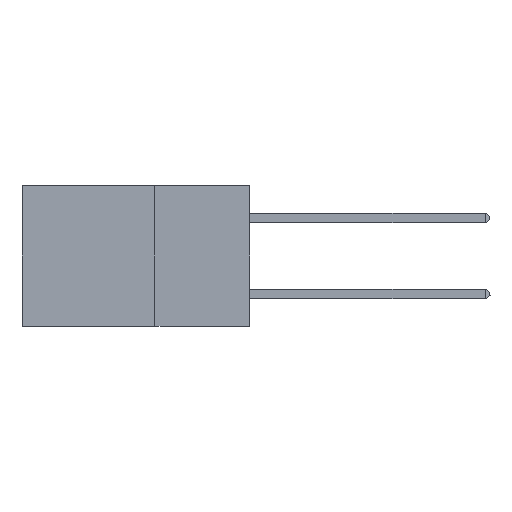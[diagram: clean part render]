
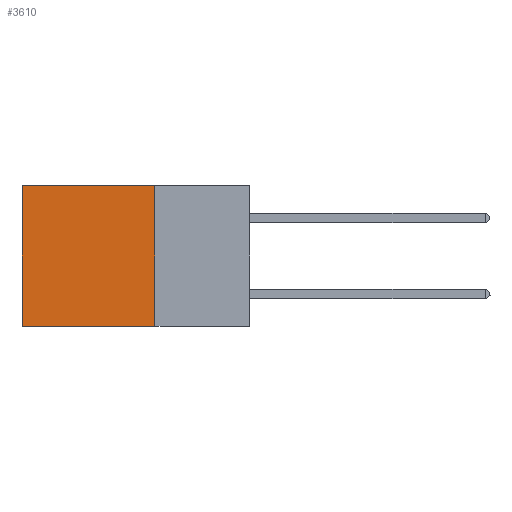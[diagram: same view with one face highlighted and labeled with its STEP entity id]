
A CAD part, left-side view. The second image highlights one B-rep face of the part: STEP entity #3610.
In plain terms, the highlighted planar face has unit normal (-1, 0, 0).
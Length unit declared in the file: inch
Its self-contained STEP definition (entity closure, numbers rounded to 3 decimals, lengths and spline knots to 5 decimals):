
#466 = CARTESIAN_POINT ( 'NONE',  ( 0.2875, 0.25, 0. ) ) ;
#864 = CARTESIAN_POINT ( 'NONE',  ( 0.2875, 0.25, 0. ) ) ;
#1117 = VECTOR ( 'NONE', #8852, 39.37008 ) ;
#1227 = CARTESIAN_POINT ( 'NONE',  ( 0.2875, 0.25, 0. ) ) ;
#1508 = DIRECTION ( 'NONE',  ( 0., 0., -1. ) ) ;
#2467 = VERTEX_POINT ( 'NONE', #14720 ) ;
#3610 = ADVANCED_FACE ( 'NONE', ( #17761 ), #21781, .F. ) ;
#3894 = VECTOR ( 'NONE', #4807, 39.37008 ) ;
#4807 = DIRECTION ( 'NONE',  ( 0., 1., 0. ) ) ;
#6198 = DIRECTION ( 'NONE',  ( 0., 0., -1. ) ) ;
#6285 = LINE ( 'NONE', #6545, #14133 ) ;
#6545 = CARTESIAN_POINT ( 'NONE',  ( 0.2875, 0.6, 0. ) ) ;
#7256 = ORIENTED_EDGE ( 'NONE', *, *, #13277, .T. ) ;
#7293 = VERTEX_POINT ( 'NONE', #466 ) ;
#8146 = ORIENTED_EDGE ( 'NONE', *, *, #11430, .F. ) ;
#8852 = DIRECTION ( 'NONE',  ( 0., 1., 0. ) ) ;
#9520 = ORIENTED_EDGE ( 'NONE', *, *, #18389, .F. ) ;
#9858 = CARTESIAN_POINT ( 'NONE',  ( 0.2875, 0.25, -0.37 ) ) ;
#10130 = VECTOR ( 'NONE', #15406, 39.37008 ) ;
#11174 = DIRECTION ( 'NONE',  ( 1., 0., 0. ) ) ;
#11430 = EDGE_CURVE ( 'NONE', #2467, #13355, #16371, .T. ) ;
#12296 = VERTEX_POINT ( 'NONE', #17231 ) ;
#13277 = EDGE_CURVE ( 'NONE', #7293, #12296, #16304, .T. ) ;
#13355 = VERTEX_POINT ( 'NONE', #21874 ) ;
#14133 = VECTOR ( 'NONE', #1508, 39.37008 ) ;
#14720 = CARTESIAN_POINT ( 'NONE',  ( 0.2875, 0.25, -0.37 ) ) ;
#15386 = CARTESIAN_POINT ( 'NONE',  ( 0.2875, 0.25, 0. ) ) ;
#15406 = DIRECTION ( 'NONE',  ( 0., 0., -1. ) ) ;
#16304 = LINE ( 'NONE', #15386, #1117 ) ;
#16358 = LINE ( 'NONE', #1227, #10130 ) ;
#16371 = LINE ( 'NONE', #9858, #3894 ) ;
#17231 = CARTESIAN_POINT ( 'NONE',  ( 0.2875, 0.6, 0. ) ) ;
#17456 = ORIENTED_EDGE ( 'NONE', *, *, #17701, .T. ) ;
#17701 = EDGE_CURVE ( 'NONE', #12296, #13355, #6285, .T. ) ;
#17761 = FACE_OUTER_BOUND ( 'NONE', #20917, .T. ) ;
#18389 = EDGE_CURVE ( 'NONE', #7293, #2467, #16358, .T. ) ;
#19332 = AXIS2_PLACEMENT_3D ( 'NONE', #864, #11174, #6198 ) ;
#20917 = EDGE_LOOP ( 'NONE', ( #17456, #8146, #9520, #7256 ) ) ;
#21781 = PLANE ( 'NONE',  #19332 ) ;
#21874 = CARTESIAN_POINT ( 'NONE',  ( 0.2875, 0.6, -0.37 ) ) ;
